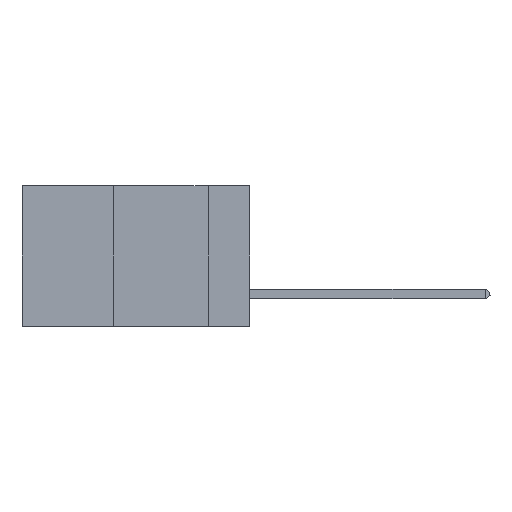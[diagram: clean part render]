
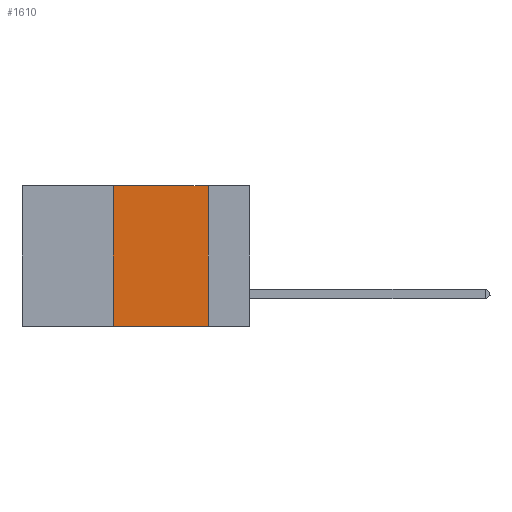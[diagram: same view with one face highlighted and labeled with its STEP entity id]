
A CAD part, left-side view. The second image highlights one B-rep face of the part: STEP entity #1610.
In plain terms, the highlighted planar face has unit normal (-1, 0, 0).
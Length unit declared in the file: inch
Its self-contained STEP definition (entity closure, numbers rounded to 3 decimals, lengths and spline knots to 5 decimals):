
#316 = ORIENTED_EDGE ( 'NONE', *, *, #9683, .F. ) ;
#336 = DIRECTION ( 'NONE',  ( 0., 0., 1. ) ) ;
#933 = LINE ( 'NONE', #9774, #3292 ) ;
#1170 = VECTOR ( 'NONE', #11544, 39.37008 ) ;
#1476 = CARTESIAN_POINT ( 'NONE',  ( 0., 0.6, 0. ) ) ;
#1610 = ADVANCED_FACE ( 'NONE', ( #8373 ), #6426, .F. ) ;
#2103 = EDGE_LOOP ( 'NONE', ( #9900, #316, #8103, #7281 ) ) ;
#2464 = CARTESIAN_POINT ( 'NONE',  ( 0., 0.11, 0. ) ) ;
#3292 = VECTOR ( 'NONE', #336, 39.37008 ) ;
#3303 = CARTESIAN_POINT ( 'NONE',  ( 0., 0.36, -0.37 ) ) ;
#3331 = EDGE_CURVE ( 'NONE', #3681, #8734, #12820, .T. ) ;
#3681 = VERTEX_POINT ( 'NONE', #5542 ) ;
#3690 = LINE ( 'NONE', #10710, #1170 ) ;
#4346 = VERTEX_POINT ( 'NONE', #3303 ) ;
#4567 = DIRECTION ( 'NONE',  ( 0., 0., -1. ) ) ;
#4663 = DIRECTION ( 'NONE',  ( 0., -1., 0. ) ) ;
#5542 = CARTESIAN_POINT ( 'NONE',  ( 0., 0.11, 0. ) ) ;
#6426 = PLANE ( 'NONE',  #12914 ) ;
#6489 = VECTOR ( 'NONE', #4567, 39.37008 ) ;
#7281 = ORIENTED_EDGE ( 'NONE', *, *, #8406, .T. ) ;
#7385 = CARTESIAN_POINT ( 'NONE',  ( 0., 0.11, -0.37 ) ) ;
#8103 = ORIENTED_EDGE ( 'NONE', *, *, #13630, .F. ) ;
#8373 = FACE_OUTER_BOUND ( 'NONE', #2103, .T. ) ;
#8406 = EDGE_CURVE ( 'NONE', #4346, #8734, #3690, .T. ) ;
#8734 = VERTEX_POINT ( 'NONE', #7385 ) ;
#9185 = DIRECTION ( 'NONE',  ( 0., 0., -1. ) ) ;
#9683 = EDGE_CURVE ( 'NONE', #13200, #3681, #10663, .T. ) ;
#9774 = CARTESIAN_POINT ( 'NONE',  ( 0., 0.36, 0. ) ) ;
#9900 = ORIENTED_EDGE ( 'NONE', *, *, #3331, .F. ) ;
#10383 = DIRECTION ( 'NONE',  ( 1., 0., 0. ) ) ;
#10663 = LINE ( 'NONE', #1476, #12444 ) ;
#10710 = CARTESIAN_POINT ( 'NONE',  ( 0., 0.6, -0.37 ) ) ;
#11544 = DIRECTION ( 'NONE',  ( 0., -1., 0. ) ) ;
#12444 = VECTOR ( 'NONE', #4663, 39.37008 ) ;
#12820 = LINE ( 'NONE', #2464, #6489 ) ;
#12914 = AXIS2_PLACEMENT_3D ( 'NONE', #13517, #10383, #9185 ) ;
#13200 = VERTEX_POINT ( 'NONE', #13606 ) ;
#13517 = CARTESIAN_POINT ( 'NONE',  ( 0., 0.6, 0. ) ) ;
#13606 = CARTESIAN_POINT ( 'NONE',  ( 0., 0.36, 0. ) ) ;
#13630 = EDGE_CURVE ( 'NONE', #4346, #13200, #933, .T. ) ;
